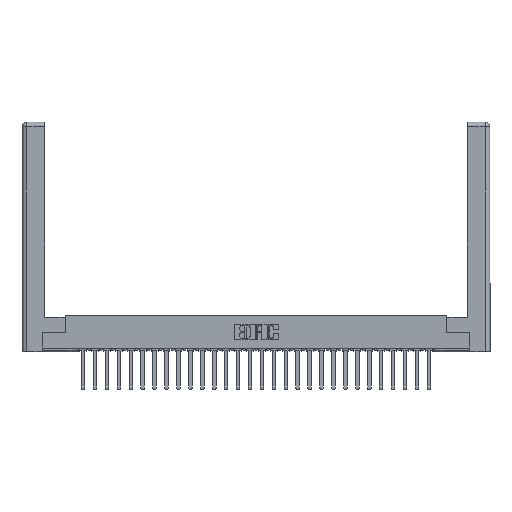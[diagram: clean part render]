
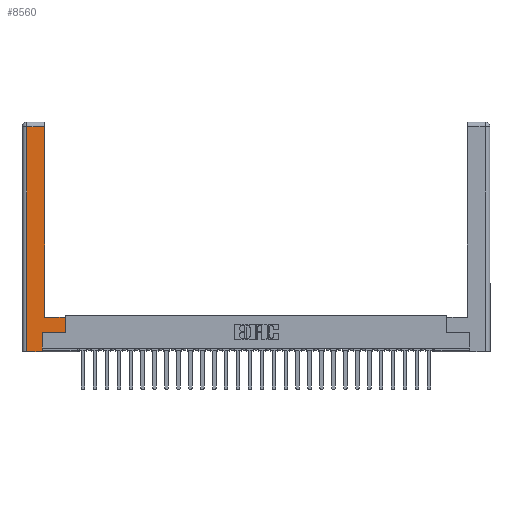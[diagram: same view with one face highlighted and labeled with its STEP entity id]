
A CAD part, top view. The second image highlights one B-rep face of the part: STEP entity #8560.
In plain terms, the highlighted planar face has unit normal (0, 0, 1).
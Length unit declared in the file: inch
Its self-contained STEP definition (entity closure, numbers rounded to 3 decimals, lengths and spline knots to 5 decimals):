
#54 = EDGE_CURVE ( 'NONE', #14553, #15097, #13619, .T. ) ;
#1355 = DIRECTION ( 'NONE',  ( -1., 0., 0. ) ) ;
#2091 = AXIS2_PLACEMENT_3D ( 'NONE', #24729, #5549, #1355 ) ;
#2691 = VECTOR ( 'NONE', #7049, 39.37008 ) ;
#2759 = CARTESIAN_POINT ( 'NONE',  ( 0.265, 0., 0. ) ) ;
#2768 = ORIENTED_EDGE ( 'NONE', *, *, #54, .T. ) ;
#2904 = ORIENTED_EDGE ( 'NONE', *, *, #14208, .T. ) ;
#2970 = CARTESIAN_POINT ( 'NONE',  ( 0.295, 3., 0. ) ) ;
#3993 = CARTESIAN_POINT ( 'NONE',  ( 0.265, 0.245, 0. ) ) ;
#4064 = EDGE_CURVE ( 'NONE', #17988, #20214, #25545, .T. ) ;
#5044 = DIRECTION ( 'NONE',  ( 0., 1., 0. ) ) ;
#5507 = CARTESIAN_POINT ( 'NONE',  ( 0.565, 0.45, 0. ) ) ;
#5549 = DIRECTION ( 'NONE',  ( 0., 0., -1. ) ) ;
#5827 = VERTEX_POINT ( 'NONE', #2759 ) ;
#5870 = ORIENTED_EDGE ( 'NONE', *, *, #27187, .T. ) ;
#6556 = ORIENTED_EDGE ( 'NONE', *, *, #6841, .T. ) ;
#6831 = VERTEX_POINT ( 'NONE', #24162 ) ;
#6841 = EDGE_CURVE ( 'NONE', #20214, #13871, #16747, .T. ) ;
#7049 = DIRECTION ( 'NONE',  ( 0., 1., 0. ) ) ;
#7426 = VECTOR ( 'NONE', #29353, 39.37008 ) ;
#7747 = LINE ( 'NONE', #12085, #22403 ) ;
#8560 = ADVANCED_FACE ( 'NONE', ( #17624 ), #22565, .F. ) ;
#9023 = CARTESIAN_POINT ( 'NONE',  ( 0.295, 2.94, 0. ) ) ;
#9120 = EDGE_LOOP ( 'NONE', ( #6556, #2904, #2768, #13954, #5870, #20910, #15371, #13124 ) ) ;
#10949 = CARTESIAN_POINT ( 'NONE',  ( 0.0615, 2.94, 0. ) ) ;
#12043 = VERTEX_POINT ( 'NONE', #18468 ) ;
#12085 = CARTESIAN_POINT ( 'NONE',  ( 0.565, 0.245, 0. ) ) ;
#12237 = DIRECTION ( 'NONE',  ( 1., 0., 0. ) ) ;
#12977 = CARTESIAN_POINT ( 'NONE',  ( 0.265, 0., 0. ) ) ;
#13124 = ORIENTED_EDGE ( 'NONE', *, *, #4064, .T. ) ;
#13619 = LINE ( 'NONE', #24900, #17519 ) ;
#13871 = VERTEX_POINT ( 'NONE', #9023 ) ;
#13954 = ORIENTED_EDGE ( 'NONE', *, *, #20915, .T. ) ;
#14208 = EDGE_CURVE ( 'NONE', #13871, #14553, #27809, .T. ) ;
#14421 = EDGE_CURVE ( 'NONE', #12043, #17988, #16983, .T. ) ;
#14553 = VERTEX_POINT ( 'NONE', #24536 ) ;
#15097 = VERTEX_POINT ( 'NONE', #25695 ) ;
#15371 = ORIENTED_EDGE ( 'NONE', *, *, #14421, .T. ) ;
#15961 = DIRECTION ( 'NONE',  ( -1., 0., 0. ) ) ;
#16633 = VECTOR ( 'NONE', #27351, 39.37008 ) ;
#16747 = LINE ( 'NONE', #2970, #29738 ) ;
#16983 = LINE ( 'NONE', #5507, #23596 ) ;
#17519 = VECTOR ( 'NONE', #23048, 39.37008 ) ;
#17624 = FACE_OUTER_BOUND ( 'NONE', #9120, .T. ) ;
#17988 = VERTEX_POINT ( 'NONE', #27563 ) ;
#18100 = LINE ( 'NONE', #3993, #2691 ) ;
#18468 = CARTESIAN_POINT ( 'NONE',  ( 0.565, 0.245, 0. ) ) ;
#20214 = VERTEX_POINT ( 'NONE', #24985 ) ;
#20910 = ORIENTED_EDGE ( 'NONE', *, *, #25653, .T. ) ;
#20915 = EDGE_CURVE ( 'NONE', #15097, #5827, #29513, .T. ) ;
#21856 = DIRECTION ( 'NONE',  ( 0., 1., 0. ) ) ;
#22403 = VECTOR ( 'NONE', #12237, 39.37008 ) ;
#22565 = PLANE ( 'NONE',  #2091 ) ;
#23048 = DIRECTION ( 'NONE',  ( 0., -1., 0. ) ) ;
#23596 = VECTOR ( 'NONE', #5044, 39.37008 ) ;
#24162 = CARTESIAN_POINT ( 'NONE',  ( 0.265, 0.245, 0. ) ) ;
#24536 = CARTESIAN_POINT ( 'NONE',  ( 0.0615, 2.94, 0. ) ) ;
#24729 = CARTESIAN_POINT ( 'NONE',  ( 0., 0., 0. ) ) ;
#24900 = CARTESIAN_POINT ( 'NONE',  ( 0.0615, 0., 0. ) ) ;
#24985 = CARTESIAN_POINT ( 'NONE',  ( 0.295, 0.45, 0. ) ) ;
#25545 = LINE ( 'NONE', #30183, #27052 ) ;
#25653 = EDGE_CURVE ( 'NONE', #6831, #12043, #7747, .T. ) ;
#25695 = CARTESIAN_POINT ( 'NONE',  ( 0.0615, 0., 0. ) ) ;
#27052 = VECTOR ( 'NONE', #15961, 39.37008 ) ;
#27187 = EDGE_CURVE ( 'NONE', #5827, #6831, #18100, .T. ) ;
#27351 = DIRECTION ( 'NONE',  ( -1., 0., 0. ) ) ;
#27563 = CARTESIAN_POINT ( 'NONE',  ( 0.565, 0.45, 0. ) ) ;
#27809 = LINE ( 'NONE', #10949, #16633 ) ;
#29353 = DIRECTION ( 'NONE',  ( 1., 0., 0. ) ) ;
#29513 = LINE ( 'NONE', #12977, #7426 ) ;
#29738 = VECTOR ( 'NONE', #21856, 39.37008 ) ;
#30183 = CARTESIAN_POINT ( 'NONE',  ( 0.295, 0.45, 0. ) ) ;
